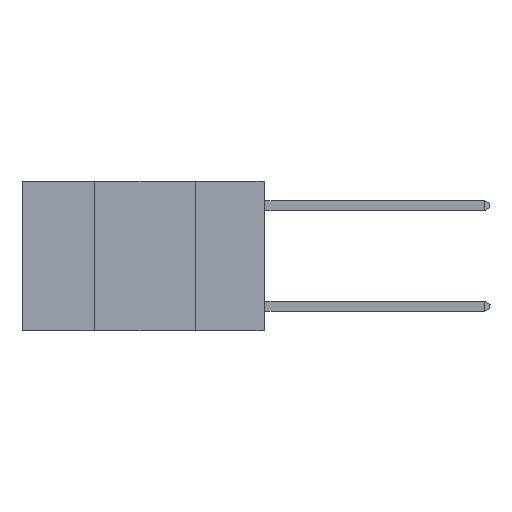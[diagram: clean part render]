
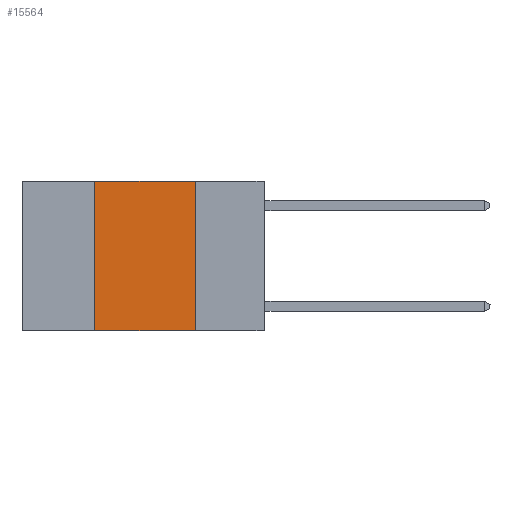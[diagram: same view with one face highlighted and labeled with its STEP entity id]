
A CAD part, left-side view. The second image highlights one B-rep face of the part: STEP entity #15564.
In plain terms, the highlighted planar face has unit normal (-1, 0, 0).
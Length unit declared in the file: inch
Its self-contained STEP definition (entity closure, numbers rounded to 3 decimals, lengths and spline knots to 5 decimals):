
#1046 = PLANE ( 'NONE',  #4935 ) ;
#1617 = VERTEX_POINT ( 'NONE', #20120 ) ;
#1646 = CARTESIAN_POINT ( 'NONE',  ( 0., 0.17, 0. ) ) ;
#1994 = EDGE_CURVE ( 'NONE', #2166, #1617, #28230, .T. ) ;
#2166 = VERTEX_POINT ( 'NONE', #1646 ) ;
#4935 = AXIS2_PLACEMENT_3D ( 'NONE', #26471, #11249, #29032 ) ;
#5487 = LINE ( 'NONE', #5844, #19791 ) ;
#5844 = CARTESIAN_POINT ( 'NONE',  ( 0., 0.42, 0. ) ) ;
#6464 = ORIENTED_EDGE ( 'NONE', *, *, #23033, .F. ) ;
#8389 = DIRECTION ( 'NONE',  ( 0., 0., 1. ) ) ;
#8560 = EDGE_CURVE ( 'NONE', #17211, #1617, #14355, .T. ) ;
#9083 = CARTESIAN_POINT ( 'NONE',  ( 0., 0.6, -0.37 ) ) ;
#10874 = VECTOR ( 'NONE', #29528, 39.37008 ) ;
#11249 = DIRECTION ( 'NONE',  ( 1., 0., 0. ) ) ;
#12477 = LINE ( 'NONE', #26971, #10874 ) ;
#13219 = ORIENTED_EDGE ( 'NONE', *, *, #31891, .F. ) ;
#14355 = LINE ( 'NONE', #9083, #21122 ) ;
#15564 = ADVANCED_FACE ( 'NONE', ( #15960 ), #1046, .F. ) ;
#15644 = EDGE_LOOP ( 'NONE', ( #31137, #6464, #13219, #19981 ) ) ;
#15960 = FACE_OUTER_BOUND ( 'NONE', #15644, .T. ) ;
#16309 = CARTESIAN_POINT ( 'NONE',  ( 0., 0.17, 0. ) ) ;
#17211 = VERTEX_POINT ( 'NONE', #23313 ) ;
#19328 = DIRECTION ( 'NONE',  ( 0., -1., 0. ) ) ;
#19791 = VECTOR ( 'NONE', #8389, 39.37008 ) ;
#19981 = ORIENTED_EDGE ( 'NONE', *, *, #8560, .T. ) ;
#20120 = CARTESIAN_POINT ( 'NONE',  ( 0., 0.17, -0.37 ) ) ;
#21122 = VECTOR ( 'NONE', #19328, 39.37008 ) ;
#22187 = VERTEX_POINT ( 'NONE', #28955 ) ;
#23033 = EDGE_CURVE ( 'NONE', #22187, #2166, #12477, .T. ) ;
#23313 = CARTESIAN_POINT ( 'NONE',  ( 0., 0.42, -0.37 ) ) ;
#24016 = DIRECTION ( 'NONE',  ( 0., 0., -1. ) ) ;
#25849 = VECTOR ( 'NONE', #24016, 39.37008 ) ;
#26471 = CARTESIAN_POINT ( 'NONE',  ( 0., 0.6, 0. ) ) ;
#26971 = CARTESIAN_POINT ( 'NONE',  ( 0., 0.6, 0. ) ) ;
#28230 = LINE ( 'NONE', #16309, #25849 ) ;
#28955 = CARTESIAN_POINT ( 'NONE',  ( 0., 0.42, 0. ) ) ;
#29032 = DIRECTION ( 'NONE',  ( 0., 0., -1. ) ) ;
#29528 = DIRECTION ( 'NONE',  ( 0., -1., 0. ) ) ;
#31137 = ORIENTED_EDGE ( 'NONE', *, *, #1994, .F. ) ;
#31891 = EDGE_CURVE ( 'NONE', #17211, #22187, #5487, .T. ) ;
